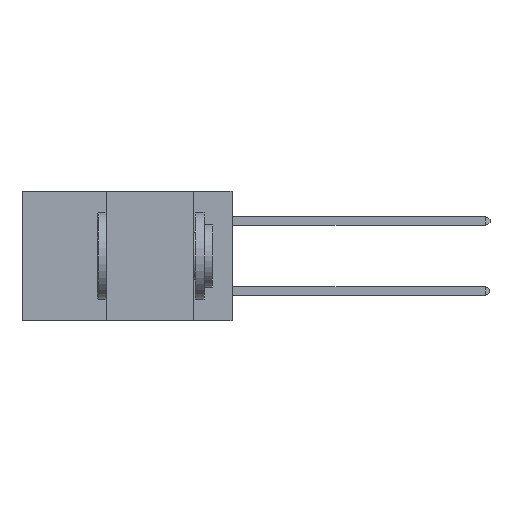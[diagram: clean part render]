
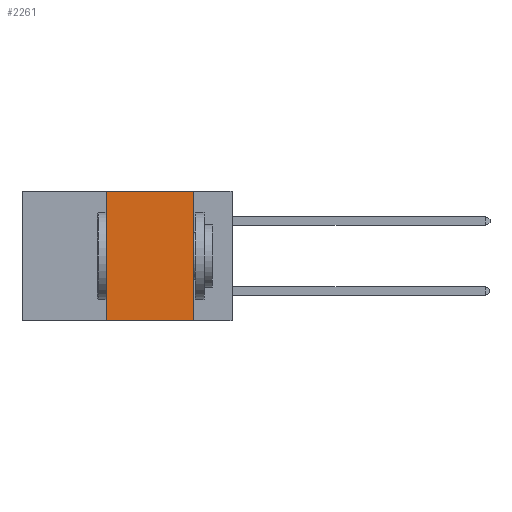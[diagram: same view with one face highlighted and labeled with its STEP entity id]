
A CAD part, left-side view. The second image highlights one B-rep face of the part: STEP entity #2261.
In plain terms, the highlighted planar face has unit normal (-1, 0, 0).
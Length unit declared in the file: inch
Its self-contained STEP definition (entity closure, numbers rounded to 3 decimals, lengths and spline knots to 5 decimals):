
#259 = EDGE_CURVE ( 'NONE', #15625, #8718, #5544, .T. ) ;
#2257 = ORIENTED_EDGE ( 'NONE', *, *, #9247, .T. ) ;
#2261 = ADVANCED_FACE ( 'NONE', ( #3701 ), #4825, .F. ) ;
#3246 = VECTOR ( 'NONE', #15663, 39.37008 ) ;
#3403 = ORIENTED_EDGE ( 'NONE', *, *, #15311, .F. ) ;
#3701 = FACE_OUTER_BOUND ( 'NONE', #3959, .T. ) ;
#3831 = CARTESIAN_POINT ( 'NONE',  ( 0., 0.11, -0.37 ) ) ;
#3959 = EDGE_LOOP ( 'NONE', ( #16600, #3403, #16211, #2257 ) ) ;
#4052 = VECTOR ( 'NONE', #12316, 39.37008 ) ;
#4825 = PLANE ( 'NONE',  #13389 ) ;
#5544 = LINE ( 'NONE', #6861, #6013 ) ;
#5786 = DIRECTION ( 'NONE',  ( 0., 0., -1. ) ) ;
#5821 = LINE ( 'NONE', #11650, #12448 ) ;
#5887 = CARTESIAN_POINT ( 'NONE',  ( 0., 0.11, 0. ) ) ;
#6013 = VECTOR ( 'NONE', #6873, 39.37008 ) ;
#6502 = CARTESIAN_POINT ( 'NONE',  ( 0., 0.36, 0. ) ) ;
#6861 = CARTESIAN_POINT ( 'NONE',  ( 0., 0.11, 0. ) ) ;
#6873 = DIRECTION ( 'NONE',  ( 0., 0., -1. ) ) ;
#7664 = DIRECTION ( 'NONE',  ( 1., 0., 0. ) ) ;
#8718 = VERTEX_POINT ( 'NONE', #3831 ) ;
#8906 = EDGE_CURVE ( 'NONE', #14699, #13809, #14658, .T. ) ;
#9247 = EDGE_CURVE ( 'NONE', #14699, #8718, #5821, .T. ) ;
#9754 = CARTESIAN_POINT ( 'NONE',  ( 0., 0.36, 0. ) ) ;
#10360 = CARTESIAN_POINT ( 'NONE',  ( 0., 0.36, -0.37 ) ) ;
#11650 = CARTESIAN_POINT ( 'NONE',  ( 0., 0.6, -0.37 ) ) ;
#12316 = DIRECTION ( 'NONE',  ( 0., 0., 1. ) ) ;
#12448 = VECTOR ( 'NONE', #14127, 39.37008 ) ;
#13389 = AXIS2_PLACEMENT_3D ( 'NONE', #14336, #7664, #5786 ) ;
#13809 = VERTEX_POINT ( 'NONE', #6502 ) ;
#13924 = LINE ( 'NONE', #14376, #3246 ) ;
#14127 = DIRECTION ( 'NONE',  ( 0., -1., 0. ) ) ;
#14336 = CARTESIAN_POINT ( 'NONE',  ( 0., 0.6, 0. ) ) ;
#14376 = CARTESIAN_POINT ( 'NONE',  ( 0., 0.6, 0. ) ) ;
#14658 = LINE ( 'NONE', #9754, #4052 ) ;
#14699 = VERTEX_POINT ( 'NONE', #10360 ) ;
#15311 = EDGE_CURVE ( 'NONE', #13809, #15625, #13924, .T. ) ;
#15625 = VERTEX_POINT ( 'NONE', #5887 ) ;
#15663 = DIRECTION ( 'NONE',  ( 0., -1., 0. ) ) ;
#16211 = ORIENTED_EDGE ( 'NONE', *, *, #8906, .F. ) ;
#16600 = ORIENTED_EDGE ( 'NONE', *, *, #259, .F. ) ;
